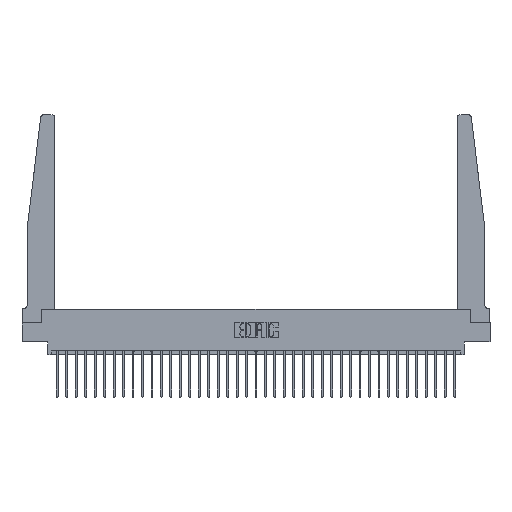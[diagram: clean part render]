
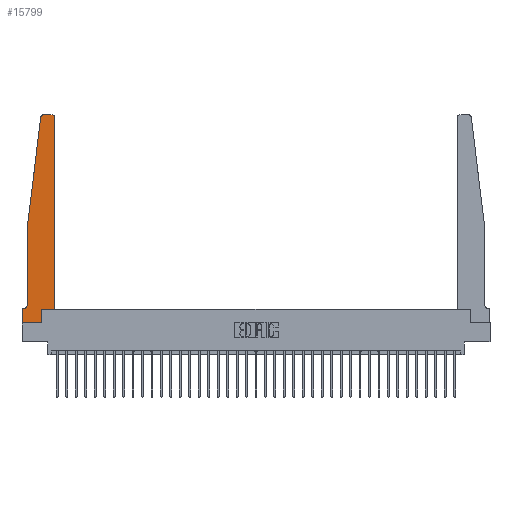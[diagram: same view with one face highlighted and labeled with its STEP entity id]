
A CAD part, top view. The second image highlights one B-rep face of the part: STEP entity #15799.
In plain terms, the highlighted planar face has unit normal (0, 0, 1).
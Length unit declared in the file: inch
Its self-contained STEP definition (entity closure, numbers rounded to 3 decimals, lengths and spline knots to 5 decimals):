
#909 = ORIENTED_EDGE ( 'NONE', *, *, #23232, .T. ) ;
#922 = DIRECTION ( 'NONE',  ( 0., 0., 1. ) ) ;
#994 = CARTESIAN_POINT ( 'NONE',  ( 0., 0., 0.37 ) ) ;
#1021 = AXIS2_PLACEMENT_3D ( 'NONE', #31263, #21613, #18431 ) ;
#1150 = CARTESIAN_POINT ( 'NONE',  ( 0., 0.1875, 0.37 ) ) ;
#1321 = EDGE_LOOP ( 'NONE', ( #17949, #32977, #2301, #24823, #25564, #26939, #909, #13476, #10828, #14409, #4129, #8007 ) ) ;
#1562 = LINE ( 'NONE', #24298, #16011 ) ;
#2301 = ORIENTED_EDGE ( 'NONE', *, *, #4552, .T. ) ;
#2361 = AXIS2_PLACEMENT_3D ( 'NONE', #12887, #20640, #4649 ) ;
#2510 = EDGE_CURVE ( 'NONE', #16449, #17714, #31447, .T. ) ;
#2518 = CARTESIAN_POINT ( 'NONE',  ( 0.2605, 0.18, 0.37 ) ) ;
#2795 = PLANE ( 'NONE',  #2361 ) ;
#3017 = CARTESIAN_POINT ( 'NONE',  ( 0.425, 0.18, 0.37 ) ) ;
#3891 = LINE ( 'NONE', #32546, #15555 ) ;
#4129 = ORIENTED_EDGE ( 'NONE', *, *, #2510, .T. ) ;
#4291 = CIRCLE ( 'NONE', #23132, 0.03 ) ;
#4299 = CARTESIAN_POINT ( 'NONE',  ( 0.27653, 2.75, 0.37 ) ) ;
#4493 = EDGE_CURVE ( 'NONE', #15795, #21591, #1562, .T. ) ;
#4552 = EDGE_CURVE ( 'NONE', #19811, #15083, #7090, .T. ) ;
#4649 = DIRECTION ( 'NONE',  ( 1., 0., 0. ) ) ;
#5510 = VERTEX_POINT ( 'NONE', #1150 ) ;
#6836 = EDGE_CURVE ( 'NONE', #19844, #27750, #21487, .T. ) ;
#7090 = LINE ( 'NONE', #14339, #31098 ) ;
#7431 = CARTESIAN_POINT ( 'NONE',  ( 0.015, 0.1875, 0.37 ) ) ;
#7719 = LINE ( 'NONE', #2518, #16243 ) ;
#8007 = ORIENTED_EDGE ( 'NONE', *, *, #20070, .T. ) ;
#8953 = DIRECTION ( 'NONE',  ( -1., 0., 0. ) ) ;
#9179 = EDGE_CURVE ( 'NONE', #21591, #19811, #4291, .T. ) ;
#9277 = CARTESIAN_POINT ( 'NONE',  ( 0.425, 2.72, 0.37 ) ) ;
#9293 = VERTEX_POINT ( 'NONE', #24810 ) ;
#10828 = ORIENTED_EDGE ( 'NONE', *, *, #11685, .T. ) ;
#11685 = EDGE_CURVE ( 'NONE', #9293, #32313, #7719, .T. ) ;
#11770 = EDGE_CURVE ( 'NONE', #32313, #16449, #18340, .T. ) ;
#12438 = VECTOR ( 'NONE', #15733, 39.37008 ) ;
#12774 = DIRECTION ( 'NONE',  ( 0., 1., 0. ) ) ;
#12887 = CARTESIAN_POINT ( 'NONE',  ( 0., 0.1875, 0.37 ) ) ;
#13291 = DIRECTION ( 'NONE',  ( 0., 0., -1. ) ) ;
#13476 = ORIENTED_EDGE ( 'NONE', *, *, #29932, .T. ) ;
#13705 = LINE ( 'NONE', #23987, #31860 ) ;
#14339 = CARTESIAN_POINT ( 'NONE',  ( 0.065, 1.25, 0.37 ) ) ;
#14409 = ORIENTED_EDGE ( 'NONE', *, *, #11770, .T. ) ;
#14454 = CARTESIAN_POINT ( 'NONE',  ( 0.2605, 0.18, 0.37 ) ) ;
#15083 = VERTEX_POINT ( 'NONE', #19559 ) ;
#15555 = VECTOR ( 'NONE', #17177, 39.37008 ) ;
#15670 = VECTOR ( 'NONE', #32500, 39.37008 ) ;
#15717 = VECTOR ( 'NONE', #26585, 39.37008 ) ;
#15733 = DIRECTION ( 'NONE',  ( 0., -1., 0. ) ) ;
#15795 = VERTEX_POINT ( 'NONE', #25364 ) ;
#15799 = ADVANCED_FACE ( 'NONE', ( #30441 ), #2795, .T. ) ;
#16002 = CIRCLE ( 'NONE', #1021, 0.03 ) ;
#16011 = VECTOR ( 'NONE', #8953, 39.37008 ) ;
#16243 = VECTOR ( 'NONE', #12774, 39.37008 ) ;
#16449 = VERTEX_POINT ( 'NONE', #28875 ) ;
#17177 = DIRECTION ( 'NONE',  ( -1., 0., 0. ) ) ;
#17529 = VECTOR ( 'NONE', #26700, 39.37008 ) ;
#17714 = VERTEX_POINT ( 'NONE', #9277 ) ;
#17949 = ORIENTED_EDGE ( 'NONE', *, *, #4493, .T. ) ;
#18340 = LINE ( 'NONE', #3017, #15717 ) ;
#18431 = DIRECTION ( 'NONE',  ( 1., 0., 0. ) ) ;
#19434 = DIRECTION ( 'NONE',  ( 1., 0., 0. ) ) ;
#19559 = CARTESIAN_POINT ( 'NONE',  ( 0.065, 1.25, 0.37 ) ) ;
#19811 = VERTEX_POINT ( 'NONE', #27596 ) ;
#19837 = CARTESIAN_POINT ( 'NONE',  ( 0.065, 0.2375, 0.37 ) ) ;
#19844 = VERTEX_POINT ( 'NONE', #19837 ) ;
#20070 = EDGE_CURVE ( 'NONE', #17714, #15795, #16002, .T. ) ;
#20556 = EDGE_CURVE ( 'NONE', #27750, #5510, #3891, .T. ) ;
#20640 = DIRECTION ( 'NONE',  ( 0., 0., 1. ) ) ;
#20876 = DIRECTION ( 'NONE',  ( -1., 0., 0. ) ) ;
#21447 = DIRECTION ( 'NONE',  ( 0., -1., 0. ) ) ;
#21487 = CIRCLE ( 'NONE', #27425, 0.05 ) ;
#21591 = VERTEX_POINT ( 'NONE', #4299 ) ;
#21613 = DIRECTION ( 'NONE',  ( 0., 0., 1. ) ) ;
#23132 = AXIS2_PLACEMENT_3D ( 'NONE', #31931, #922, #19434 ) ;
#23232 = EDGE_CURVE ( 'NONE', #5510, #26213, #13705, .T. ) ;
#23987 = CARTESIAN_POINT ( 'NONE',  ( 0., 0., 0.37 ) ) ;
#24298 = CARTESIAN_POINT ( 'NONE',  ( 0.25, 2.75, 0.37 ) ) ;
#24810 = CARTESIAN_POINT ( 'NONE',  ( 0.2605, 0., 0.37 ) ) ;
#24823 = ORIENTED_EDGE ( 'NONE', *, *, #30687, .T. ) ;
#24950 = DIRECTION ( 'NONE',  ( -0.122, -0.992, 0. ) ) ;
#25364 = CARTESIAN_POINT ( 'NONE',  ( 0.395, 2.75, 0.37 ) ) ;
#25564 = ORIENTED_EDGE ( 'NONE', *, *, #6836, .T. ) ;
#25849 = LINE ( 'NONE', #26020, #12438 ) ;
#26020 = CARTESIAN_POINT ( 'NONE',  ( 0.065, 1.25, 0.37 ) ) ;
#26206 = CARTESIAN_POINT ( 'NONE',  ( 0.425, 0.18, 0.37 ) ) ;
#26213 = VERTEX_POINT ( 'NONE', #31891 ) ;
#26585 = DIRECTION ( 'NONE',  ( 1., 0., 0. ) ) ;
#26700 = DIRECTION ( 'NONE',  ( 0., 1., 0. ) ) ;
#26939 = ORIENTED_EDGE ( 'NONE', *, *, #20556, .T. ) ;
#27425 = AXIS2_PLACEMENT_3D ( 'NONE', #31015, #13291, #20876 ) ;
#27596 = CARTESIAN_POINT ( 'NONE',  ( 0.24675, 2.72367, 0.37 ) ) ;
#27750 = VERTEX_POINT ( 'NONE', #7431 ) ;
#28875 = CARTESIAN_POINT ( 'NONE',  ( 0.425, 0.18, 0.37 ) ) ;
#29932 = EDGE_CURVE ( 'NONE', #26213, #9293, #29964, .T. ) ;
#29964 = LINE ( 'NONE', #994, #15670 ) ;
#30441 = FACE_OUTER_BOUND ( 'NONE', #1321, .T. ) ;
#30687 = EDGE_CURVE ( 'NONE', #15083, #19844, #25849, .T. ) ;
#31015 = CARTESIAN_POINT ( 'NONE',  ( 0.015, 0.2375, 0.37 ) ) ;
#31098 = VECTOR ( 'NONE', #24950, 39.37008 ) ;
#31263 = CARTESIAN_POINT ( 'NONE',  ( 0.395, 2.72, 0.37 ) ) ;
#31447 = LINE ( 'NONE', #26206, #17529 ) ;
#31860 = VECTOR ( 'NONE', #21447, 39.37008 ) ;
#31891 = CARTESIAN_POINT ( 'NONE',  ( 0., 0., 0.37 ) ) ;
#31931 = CARTESIAN_POINT ( 'NONE',  ( 0.27653, 2.72, 0.37 ) ) ;
#32313 = VERTEX_POINT ( 'NONE', #14454 ) ;
#32500 = DIRECTION ( 'NONE',  ( 1., 0., 0. ) ) ;
#32546 = CARTESIAN_POINT ( 'NONE',  ( 0.065, 0.1875, 0.37 ) ) ;
#32977 = ORIENTED_EDGE ( 'NONE', *, *, #9179, .T. ) ;
